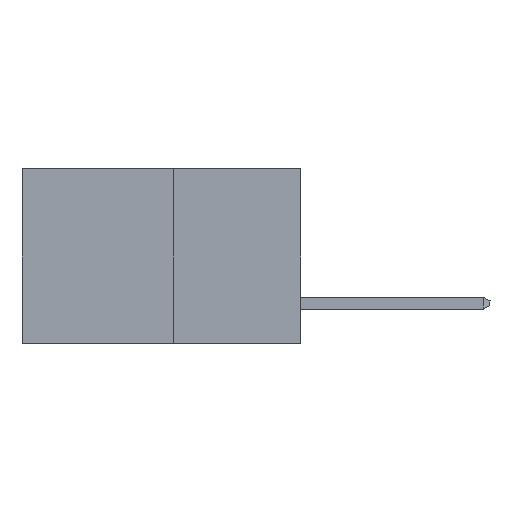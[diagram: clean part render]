
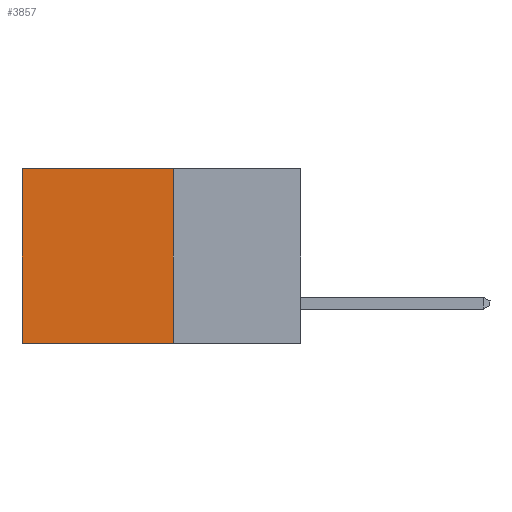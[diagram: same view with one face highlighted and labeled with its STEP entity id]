
A CAD part, left-side view. The second image highlights one B-rep face of the part: STEP entity #3857.
In plain terms, the highlighted planar face has unit normal (-1, 0, 0).
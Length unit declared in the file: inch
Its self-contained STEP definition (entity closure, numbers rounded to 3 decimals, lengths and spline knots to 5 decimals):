
#149 = EDGE_CURVE ( 'NONE', #8361, #2988, #9096, .T. ) ;
#286 = ORIENTED_EDGE ( 'NONE', *, *, #8950, .T. ) ;
#527 = ORIENTED_EDGE ( 'NONE', *, *, #10073, .T. ) ;
#1247 = VECTOR ( 'NONE', #8888, 39.37008 ) ;
#2176 = LINE ( 'NONE', #6919, #9179 ) ;
#2396 = EDGE_CURVE ( 'NONE', #2541, #8361, #2176, .T. ) ;
#2541 = VERTEX_POINT ( 'NONE', #3158 ) ;
#2988 = VERTEX_POINT ( 'NONE', #11226 ) ;
#3158 = CARTESIAN_POINT ( 'NONE',  ( 0.277, 0.27, 0. ) ) ;
#3550 = FACE_OUTER_BOUND ( 'NONE', #9073, .T. ) ;
#3857 = ADVANCED_FACE ( 'NONE', ( #3550 ), #8585, .F. ) ;
#4836 = LINE ( 'NONE', #9872, #11449 ) ;
#5914 = ORIENTED_EDGE ( 'NONE', *, *, #149, .F. ) ;
#6099 = VERTEX_POINT ( 'NONE', #11624 ) ;
#6151 = DIRECTION ( 'NONE',  ( 0., 1., 0. ) ) ;
#6748 = LINE ( 'NONE', #9044, #1247 ) ;
#6919 = CARTESIAN_POINT ( 'NONE',  ( 0.277, 0.27, -0.37 ) ) ;
#8130 = DIRECTION ( 'NONE',  ( 0., 0., -1. ) ) ;
#8287 = ORIENTED_EDGE ( 'NONE', *, *, #2396, .F. ) ;
#8361 = VERTEX_POINT ( 'NONE', #9787 ) ;
#8441 = DIRECTION ( 'NONE',  ( 0., 0., -1. ) ) ;
#8474 = DIRECTION ( 'NONE',  ( 1., 0., 0. ) ) ;
#8517 = CARTESIAN_POINT ( 'NONE',  ( 0.277, 0.27, -0.37 ) ) ;
#8585 = PLANE ( 'NONE',  #10423 ) ;
#8606 = VECTOR ( 'NONE', #6151, 39.37008 ) ;
#8888 = DIRECTION ( 'NONE',  ( 0., 0., -1. ) ) ;
#8950 = EDGE_CURVE ( 'NONE', #6099, #2988, #6748, .T. ) ;
#9028 = DIRECTION ( 'NONE',  ( 0., 1., 0. ) ) ;
#9044 = CARTESIAN_POINT ( 'NONE',  ( 0.277, 0.59, -0.37 ) ) ;
#9073 = EDGE_LOOP ( 'NONE', ( #286, #5914, #8287, #527 ) ) ;
#9096 = LINE ( 'NONE', #9774, #8606 ) ;
#9179 = VECTOR ( 'NONE', #8130, 39.37008 ) ;
#9774 = CARTESIAN_POINT ( 'NONE',  ( 0.277, 0.27, -0.37 ) ) ;
#9787 = CARTESIAN_POINT ( 'NONE',  ( 0.277, 0.27, -0.37 ) ) ;
#9872 = CARTESIAN_POINT ( 'NONE',  ( 0.277, 0.27, 0. ) ) ;
#10073 = EDGE_CURVE ( 'NONE', #2541, #6099, #4836, .T. ) ;
#10423 = AXIS2_PLACEMENT_3D ( 'NONE', #8517, #8474, #8441 ) ;
#11226 = CARTESIAN_POINT ( 'NONE',  ( 0.277, 0.59, -0.37 ) ) ;
#11449 = VECTOR ( 'NONE', #9028, 39.37008 ) ;
#11624 = CARTESIAN_POINT ( 'NONE',  ( 0.277, 0.59, 0. ) ) ;
